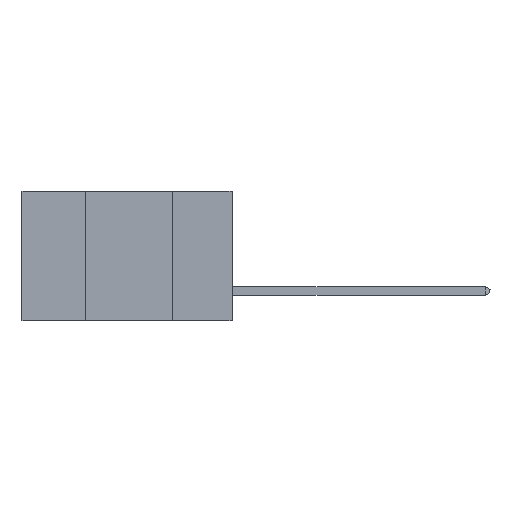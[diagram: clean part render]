
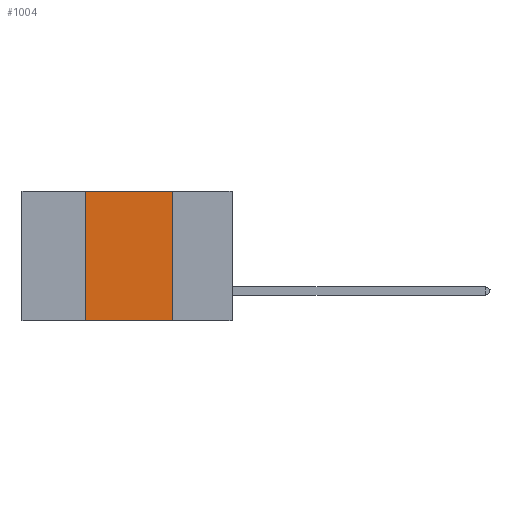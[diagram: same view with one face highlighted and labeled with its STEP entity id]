
A CAD part, left-side view. The second image highlights one B-rep face of the part: STEP entity #1004.
In plain terms, the highlighted planar face has unit normal (-1, 0, 0).
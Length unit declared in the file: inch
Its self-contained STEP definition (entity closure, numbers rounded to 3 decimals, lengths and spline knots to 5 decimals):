
#796 = LINE ( 'NONE', #8161, #18684 ) ;
#999 = LINE ( 'NONE', #6524, #15249 ) ;
#1004 = ADVANCED_FACE ( 'NONE', ( #1945 ), #17274, .F. ) ;
#1316 = VERTEX_POINT ( 'NONE', #9411 ) ;
#1429 = DIRECTION ( 'NONE',  ( 0., 0., -1. ) ) ;
#1500 = CARTESIAN_POINT ( 'NONE',  ( 0., 0.6, 0. ) ) ;
#1936 = LINE ( 'NONE', #10565, #18232 ) ;
#1945 = FACE_OUTER_BOUND ( 'NONE', #4600, .T. ) ;
#2633 = CARTESIAN_POINT ( 'NONE',  ( 0., 0.6, 0. ) ) ;
#2958 = VERTEX_POINT ( 'NONE', #16179 ) ;
#4600 = EDGE_LOOP ( 'NONE', ( #14233, #15079, #7907, #13713 ) ) ;
#6524 = CARTESIAN_POINT ( 'NONE',  ( 0., 0.6, -0.37 ) ) ;
#7414 = DIRECTION ( 'NONE',  ( 0., 0., -1. ) ) ;
#7907 = ORIENTED_EDGE ( 'NONE', *, *, #18784, .F. ) ;
#7988 = VERTEX_POINT ( 'NONE', #18483 ) ;
#8022 = EDGE_CURVE ( 'NONE', #1316, #7988, #13688, .T. ) ;
#8161 = CARTESIAN_POINT ( 'NONE',  ( 0., 0.42, 0. ) ) ;
#8573 = EDGE_CURVE ( 'NONE', #2958, #18410, #999, .T. ) ;
#8769 = EDGE_CURVE ( 'NONE', #7988, #18410, #1936, .T. ) ;
#9411 = CARTESIAN_POINT ( 'NONE',  ( 0., 0.42, 0. ) ) ;
#9418 = DIRECTION ( 'NONE',  ( 0., -1., 0. ) ) ;
#10004 = DIRECTION ( 'NONE',  ( 0., -1., 0. ) ) ;
#10211 = DIRECTION ( 'NONE',  ( 1., 0., 0. ) ) ;
#10565 = CARTESIAN_POINT ( 'NONE',  ( 0., 0.17, 0. ) ) ;
#13688 = LINE ( 'NONE', #2633, #15036 ) ;
#13713 = ORIENTED_EDGE ( 'NONE', *, *, #8573, .T. ) ;
#13858 = AXIS2_PLACEMENT_3D ( 'NONE', #1500, #10211, #1429 ) ;
#14233 = ORIENTED_EDGE ( 'NONE', *, *, #8769, .F. ) ;
#15036 = VECTOR ( 'NONE', #10004, 39.37008 ) ;
#15079 = ORIENTED_EDGE ( 'NONE', *, *, #8022, .F. ) ;
#15249 = VECTOR ( 'NONE', #9418, 39.37008 ) ;
#16179 = CARTESIAN_POINT ( 'NONE',  ( 0., 0.42, -0.37 ) ) ;
#17172 = CARTESIAN_POINT ( 'NONE',  ( 0., 0.17, -0.37 ) ) ;
#17274 = PLANE ( 'NONE',  #13858 ) ;
#18232 = VECTOR ( 'NONE', #7414, 39.37008 ) ;
#18262 = DIRECTION ( 'NONE',  ( 0., 0., 1. ) ) ;
#18410 = VERTEX_POINT ( 'NONE', #17172 ) ;
#18483 = CARTESIAN_POINT ( 'NONE',  ( 0., 0.17, 0. ) ) ;
#18684 = VECTOR ( 'NONE', #18262, 39.37008 ) ;
#18784 = EDGE_CURVE ( 'NONE', #2958, #1316, #796, .T. ) ;
